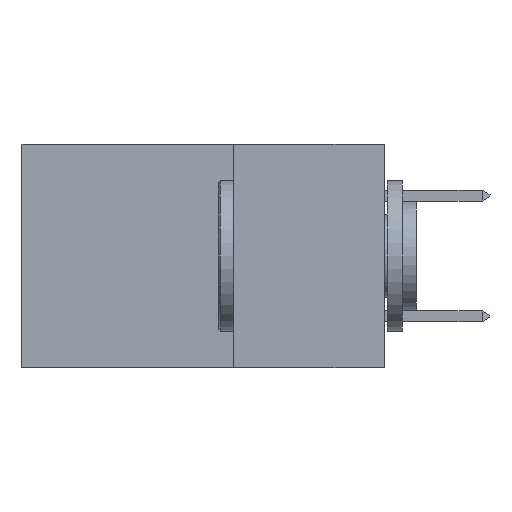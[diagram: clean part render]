
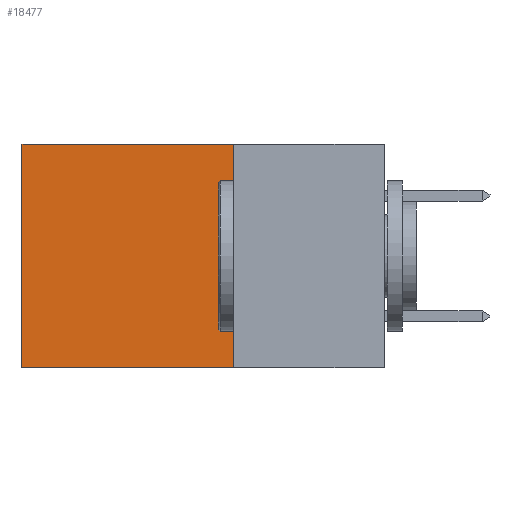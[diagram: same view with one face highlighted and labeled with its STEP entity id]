
A CAD part, left-side view. The second image highlights one B-rep face of the part: STEP entity #18477.
In plain terms, the highlighted planar face has unit normal (-1, 0, 0).
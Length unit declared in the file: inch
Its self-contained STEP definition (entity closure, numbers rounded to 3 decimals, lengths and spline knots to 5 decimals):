
#1187 = VECTOR ( 'NONE', #5259, 39.37008 ) ;
#2242 = DIRECTION ( 'NONE',  ( 0., 0., -1. ) ) ;
#2389 = LINE ( 'NONE', #14463, #17318 ) ;
#3547 = EDGE_LOOP ( 'NONE', ( #16465, #10960, #12654, #9555 ) ) ;
#3841 = PLANE ( 'NONE',  #14836 ) ;
#4039 = CARTESIAN_POINT ( 'NONE',  ( 0.2875, 0.25, -0.37 ) ) ;
#4098 = EDGE_CURVE ( 'NONE', #10931, #7199, #12789, .T. ) ;
#4545 = LINE ( 'NONE', #10965, #15581 ) ;
#5259 = DIRECTION ( 'NONE',  ( 0., 0., -1. ) ) ;
#5534 = CARTESIAN_POINT ( 'NONE',  ( 0.2875, 0.6, 0. ) ) ;
#6078 = DIRECTION ( 'NONE',  ( 0., 1., 0. ) ) ;
#6763 = CARTESIAN_POINT ( 'NONE',  ( 0.2875, 0.25, 0. ) ) ;
#7199 = VERTEX_POINT ( 'NONE', #4039 ) ;
#7313 = DIRECTION ( 'NONE',  ( 0., 1., 0. ) ) ;
#8166 = CARTESIAN_POINT ( 'NONE',  ( 0.2875, 0.6, -0.37 ) ) ;
#8212 = DIRECTION ( 'NONE',  ( 0., 0., -1. ) ) ;
#8873 = VECTOR ( 'NONE', #6078, 39.37008 ) ;
#9555 = ORIENTED_EDGE ( 'NONE', *, *, #10040, .T. ) ;
#10040 = EDGE_CURVE ( 'NONE', #10931, #16680, #12712, .T. ) ;
#10338 = CARTESIAN_POINT ( 'NONE',  ( 0.2875, 0.25, 0. ) ) ;
#10702 = FACE_OUTER_BOUND ( 'NONE', #3547, .T. ) ;
#10931 = VERTEX_POINT ( 'NONE', #10338 ) ;
#10960 = ORIENTED_EDGE ( 'NONE', *, *, #14976, .F. ) ;
#10965 = CARTESIAN_POINT ( 'NONE',  ( 0.2875, 0.6, 0. ) ) ;
#11844 = CARTESIAN_POINT ( 'NONE',  ( 0.2875, 0.25, 0. ) ) ;
#12654 = ORIENTED_EDGE ( 'NONE', *, *, #4098, .F. ) ;
#12712 = LINE ( 'NONE', #11844, #8873 ) ;
#12789 = LINE ( 'NONE', #15338, #1187 ) ;
#13285 = EDGE_CURVE ( 'NONE', #16680, #16163, #4545, .T. ) ;
#14463 = CARTESIAN_POINT ( 'NONE',  ( 0.2875, 0.25, -0.37 ) ) ;
#14836 = AXIS2_PLACEMENT_3D ( 'NONE', #6763, #16825, #8212 ) ;
#14976 = EDGE_CURVE ( 'NONE', #7199, #16163, #2389, .T. ) ;
#15338 = CARTESIAN_POINT ( 'NONE',  ( 0.2875, 0.25, 0. ) ) ;
#15581 = VECTOR ( 'NONE', #2242, 39.37008 ) ;
#16163 = VERTEX_POINT ( 'NONE', #8166 ) ;
#16465 = ORIENTED_EDGE ( 'NONE', *, *, #13285, .T. ) ;
#16680 = VERTEX_POINT ( 'NONE', #5534 ) ;
#16825 = DIRECTION ( 'NONE',  ( 1., 0., 0. ) ) ;
#17318 = VECTOR ( 'NONE', #7313, 39.37008 ) ;
#18477 = ADVANCED_FACE ( 'NONE', ( #10702 ), #3841, .F. ) ;
